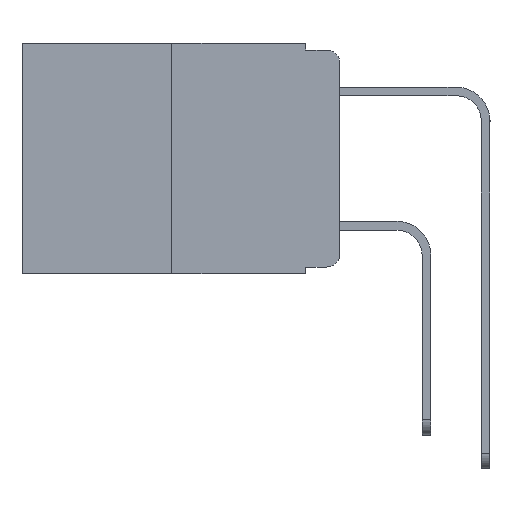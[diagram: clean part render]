
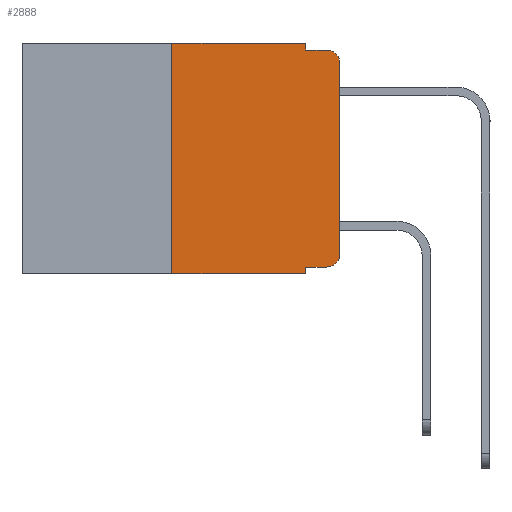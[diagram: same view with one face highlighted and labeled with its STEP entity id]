
A CAD part, left-side view. The second image highlights one B-rep face of the part: STEP entity #2888.
In plain terms, the highlighted planar face has unit normal (-1, 0, 0).
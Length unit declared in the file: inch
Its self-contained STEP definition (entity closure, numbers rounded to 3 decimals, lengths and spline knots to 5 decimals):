
#299 = CARTESIAN_POINT ( 'NONE',  ( 0., 0.051, -0.01 ) ) ;
#628 = VERTEX_POINT ( 'NONE', #18848 ) ;
#707 = ORIENTED_EDGE ( 'NONE', *, *, #17579, .F. ) ;
#896 = LINE ( 'NONE', #15712, #8910 ) ;
#1508 = CARTESIAN_POINT ( 'NONE',  ( 0., 0.473, -0.343 ) ) ;
#1512 = AXIS2_PLACEMENT_3D ( 'NONE', #16653, #6689, #18291 ) ;
#2482 = EDGE_LOOP ( 'NONE', ( #4167, #13675, #707, #5763, #3367, #3907, #21582, #13942, #5510, #19302 ) ) ;
#2656 = FACE_OUTER_BOUND ( 'NONE', #2482, .T. ) ;
#2888 = ADVANCED_FACE ( 'NONE', ( #2656 ), #21620, .F. ) ;
#3039 = VECTOR ( 'NONE', #10069, 39.37008 ) ;
#3367 = ORIENTED_EDGE ( 'NONE', *, *, #14851, .F. ) ;
#3907 = ORIENTED_EDGE ( 'NONE', *, *, #14300, .F. ) ;
#3916 = CARTESIAN_POINT ( 'NONE',  ( 0., 0.051, 0. ) ) ;
#4097 = LINE ( 'NONE', #1508, #3039 ) ;
#4167 = ORIENTED_EDGE ( 'NONE', *, *, #20851, .T. ) ;
#4291 = VERTEX_POINT ( 'NONE', #5977 ) ;
#4808 = VERTEX_POINT ( 'NONE', #16243 ) ;
#5247 = DIRECTION ( 'NONE',  ( -1., 0., 0. ) ) ;
#5440 = DIRECTION ( 'NONE',  ( 0., -1., 0. ) ) ;
#5510 = ORIENTED_EDGE ( 'NONE', *, *, #11004, .T. ) ;
#5763 = ORIENTED_EDGE ( 'NONE', *, *, #15385, .F. ) ;
#5782 = CARTESIAN_POINT ( 'NONE',  ( 0., 0.051, -0.01 ) ) ;
#5811 = VERTEX_POINT ( 'NONE', #20954 ) ;
#5977 = CARTESIAN_POINT ( 'NONE',  ( 0., 0.051, 0. ) ) ;
#5978 = LINE ( 'NONE', #12749, #18199 ) ;
#6004 = CARTESIAN_POINT ( 'NONE',  ( 0., 0.25, 0. ) ) ;
#6479 = CARTESIAN_POINT ( 'NONE',  ( 0., 0., 0. ) ) ;
#6689 = DIRECTION ( 'NONE',  ( -1., 0., 0. ) ) ;
#6802 = CARTESIAN_POINT ( 'NONE',  ( 0., 0.473, 0. ) ) ;
#7092 = VECTOR ( 'NONE', #21029, 39.37008 ) ;
#8281 = DIRECTION ( 'NONE',  ( 0., 0., 1. ) ) ;
#8411 = LINE ( 'NONE', #9265, #16677 ) ;
#8910 = VECTOR ( 'NONE', #17365, 39.37008 ) ;
#9265 = CARTESIAN_POINT ( 'NONE',  ( 0., 0.051, -0.333 ) ) ;
#9270 = CARTESIAN_POINT ( 'NONE',  ( 0., 0.051, -0.343 ) ) ;
#9303 = CARTESIAN_POINT ( 'NONE',  ( 0., 0.25, -0.343 ) ) ;
#9480 = CARTESIAN_POINT ( 'NONE',  ( 0., 0.02, -0.333 ) ) ;
#9494 = CARTESIAN_POINT ( 'NONE',  ( 0., 0.25, 0. ) ) ;
#9866 = EDGE_CURVE ( 'NONE', #14857, #5811, #10257, .T. ) ;
#9884 = CARTESIAN_POINT ( 'NONE',  ( 0., 0., -0.03 ) ) ;
#10069 = DIRECTION ( 'NONE',  ( 0., -1., 0. ) ) ;
#10257 = CIRCLE ( 'NONE', #1512, 0.02 ) ;
#11004 = EDGE_CURVE ( 'NONE', #628, #14857, #8411, .T. ) ;
#11041 = DIRECTION ( 'NONE',  ( 0., 0., -1. ) ) ;
#11284 = EDGE_CURVE ( 'NONE', #16411, #20022, #4097, .T. ) ;
#11567 = LINE ( 'NONE', #9494, #7092 ) ;
#11731 = VECTOR ( 'NONE', #5440, 39.37008 ) ;
#12122 = EDGE_CURVE ( 'NONE', #628, #20022, #12711, .T. ) ;
#12369 = DIRECTION ( 'NONE',  ( 0., 0., -1. ) ) ;
#12711 = LINE ( 'NONE', #3916, #16527 ) ;
#12749 = CARTESIAN_POINT ( 'NONE',  ( 0., 0.473, 0. ) ) ;
#13562 = VERTEX_POINT ( 'NONE', #6004 ) ;
#13675 = ORIENTED_EDGE ( 'NONE', *, *, #19771, .T. ) ;
#13803 = AXIS2_PLACEMENT_3D ( 'NONE', #15262, #5247, #16917 ) ;
#13942 = ORIENTED_EDGE ( 'NONE', *, *, #12122, .F. ) ;
#14300 = EDGE_CURVE ( 'NONE', #16411, #13562, #11567, .T. ) ;
#14851 = EDGE_CURVE ( 'NONE', #13562, #4291, #5978, .T. ) ;
#14857 = VERTEX_POINT ( 'NONE', #9480 ) ;
#15262 = CARTESIAN_POINT ( 'NONE',  ( 0., 0.02, -0.03 ) ) ;
#15385 = EDGE_CURVE ( 'NONE', #4291, #21239, #896, .T. ) ;
#15414 = DIRECTION ( 'NONE',  ( 1., 0., 0. ) ) ;
#15712 = CARTESIAN_POINT ( 'NONE',  ( 0., 0.051, 0. ) ) ;
#16243 = CARTESIAN_POINT ( 'NONE',  ( 0., 0.02, -0.01 ) ) ;
#16411 = VERTEX_POINT ( 'NONE', #9303 ) ;
#16527 = VECTOR ( 'NONE', #12369, 39.37008 ) ;
#16585 = VERTEX_POINT ( 'NONE', #9884 ) ;
#16653 = CARTESIAN_POINT ( 'NONE',  ( 0., 0.02, -0.313 ) ) ;
#16677 = VECTOR ( 'NONE', #19040, 39.37008 ) ;
#16917 = DIRECTION ( 'NONE',  ( 0., 0., -1. ) ) ;
#17143 = AXIS2_PLACEMENT_3D ( 'NONE', #6802, #15414, #11041 ) ;
#17365 = DIRECTION ( 'NONE',  ( 0., 0., -1. ) ) ;
#17579 = EDGE_CURVE ( 'NONE', #21239, #4808, #20406, .T. ) ;
#17683 = DIRECTION ( 'NONE',  ( 0., -1., 0. ) ) ;
#18199 = VECTOR ( 'NONE', #17683, 39.37008 ) ;
#18291 = DIRECTION ( 'NONE',  ( 0., 0., -1. ) ) ;
#18848 = CARTESIAN_POINT ( 'NONE',  ( 0., 0.051, -0.333 ) ) ;
#19040 = DIRECTION ( 'NONE',  ( 0., -1., 0. ) ) ;
#19168 = CIRCLE ( 'NONE', #13803, 0.02 ) ;
#19302 = ORIENTED_EDGE ( 'NONE', *, *, #9866, .T. ) ;
#19771 = EDGE_CURVE ( 'NONE', #16585, #4808, #19168, .T. ) ;
#19883 = VECTOR ( 'NONE', #8281, 39.37008 ) ;
#20022 = VERTEX_POINT ( 'NONE', #9270 ) ;
#20383 = LINE ( 'NONE', #6479, #19883 ) ;
#20406 = LINE ( 'NONE', #299, #11731 ) ;
#20851 = EDGE_CURVE ( 'NONE', #5811, #16585, #20383, .T. ) ;
#20954 = CARTESIAN_POINT ( 'NONE',  ( 0., 0., -0.313 ) ) ;
#21029 = DIRECTION ( 'NONE',  ( 0., 0., 1. ) ) ;
#21239 = VERTEX_POINT ( 'NONE', #5782 ) ;
#21582 = ORIENTED_EDGE ( 'NONE', *, *, #11284, .T. ) ;
#21620 = PLANE ( 'NONE',  #17143 ) ;
